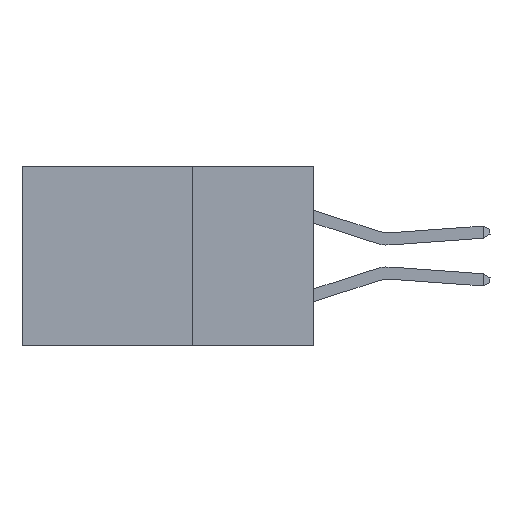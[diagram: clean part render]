
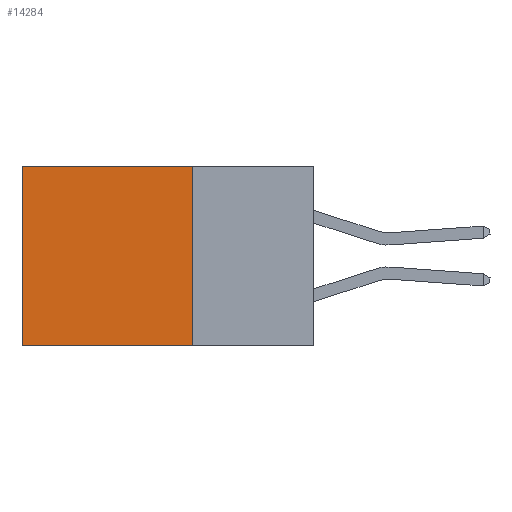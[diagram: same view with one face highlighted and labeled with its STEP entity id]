
A CAD part, left-side view. The second image highlights one B-rep face of the part: STEP entity #14284.
In plain terms, the highlighted planar face has unit normal (-1, 0, 0).
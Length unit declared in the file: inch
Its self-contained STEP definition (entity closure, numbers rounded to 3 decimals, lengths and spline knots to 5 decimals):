
#476 = CARTESIAN_POINT ( 'NONE',  ( 0.2875, 0.6, -0.37 ) ) ;
#587 = DIRECTION ( 'NONE',  ( 0., 0., -1. ) ) ;
#1412 = VERTEX_POINT ( 'NONE', #476 ) ;
#1663 = LINE ( 'NONE', #17066, #17286 ) ;
#2040 = EDGE_CURVE ( 'NONE', #21856, #9492, #16209, .T. ) ;
#3379 = CARTESIAN_POINT ( 'NONE',  ( 0.2875, 0.25, 0. ) ) ;
#3520 = CARTESIAN_POINT ( 'NONE',  ( 0.2875, 0.25, 0. ) ) ;
#3905 = LINE ( 'NONE', #3520, #5088 ) ;
#4622 = CARTESIAN_POINT ( 'NONE',  ( 0.2875, 0.25, 0. ) ) ;
#5088 = VECTOR ( 'NONE', #22272, 39.37008 ) ;
#6263 = EDGE_CURVE ( 'NONE', #9492, #1412, #20129, .T. ) ;
#8848 = DIRECTION ( 'NONE',  ( 0., 1., 0. ) ) ;
#9492 = VERTEX_POINT ( 'NONE', #22856 ) ;
#9513 = ORIENTED_EDGE ( 'NONE', *, *, #2040, .F. ) ;
#12713 = CARTESIAN_POINT ( 'NONE',  ( 0.2875, 0.25, -0.37 ) ) ;
#13737 = AXIS2_PLACEMENT_3D ( 'NONE', #3379, #22703, #24369 ) ;
#14284 = ADVANCED_FACE ( 'NONE', ( #23307 ), #14712, .F. ) ;
#14712 = PLANE ( 'NONE',  #13737 ) ;
#15439 = VECTOR ( 'NONE', #8848, 39.37008 ) ;
#15621 = VECTOR ( 'NONE', #587, 39.37008 ) ;
#16209 = LINE ( 'NONE', #4622, #15621 ) ;
#17066 = CARTESIAN_POINT ( 'NONE',  ( 0.2875, 0.6, 0. ) ) ;
#17286 = VECTOR ( 'NONE', #19036, 39.37008 ) ;
#17562 = EDGE_CURVE ( 'NONE', #21856, #18562, #3905, .T. ) ;
#17919 = CARTESIAN_POINT ( 'NONE',  ( 0.2875, 0.25, 0. ) ) ;
#18267 = ORIENTED_EDGE ( 'NONE', *, *, #22685, .T. ) ;
#18562 = VERTEX_POINT ( 'NONE', #21540 ) ;
#18954 = ORIENTED_EDGE ( 'NONE', *, *, #17562, .T. ) ;
#19036 = DIRECTION ( 'NONE',  ( 0., 0., -1. ) ) ;
#19636 = EDGE_LOOP ( 'NONE', ( #18267, #23228, #9513, #18954 ) ) ;
#20129 = LINE ( 'NONE', #12713, #15439 ) ;
#21540 = CARTESIAN_POINT ( 'NONE',  ( 0.2875, 0.6, 0. ) ) ;
#21856 = VERTEX_POINT ( 'NONE', #17919 ) ;
#22272 = DIRECTION ( 'NONE',  ( 0., 1., 0. ) ) ;
#22685 = EDGE_CURVE ( 'NONE', #18562, #1412, #1663, .T. ) ;
#22703 = DIRECTION ( 'NONE',  ( 1., 0., 0. ) ) ;
#22856 = CARTESIAN_POINT ( 'NONE',  ( 0.2875, 0.25, -0.37 ) ) ;
#23228 = ORIENTED_EDGE ( 'NONE', *, *, #6263, .F. ) ;
#23307 = FACE_OUTER_BOUND ( 'NONE', #19636, .T. ) ;
#24369 = DIRECTION ( 'NONE',  ( 0., 0., -1. ) ) ;
